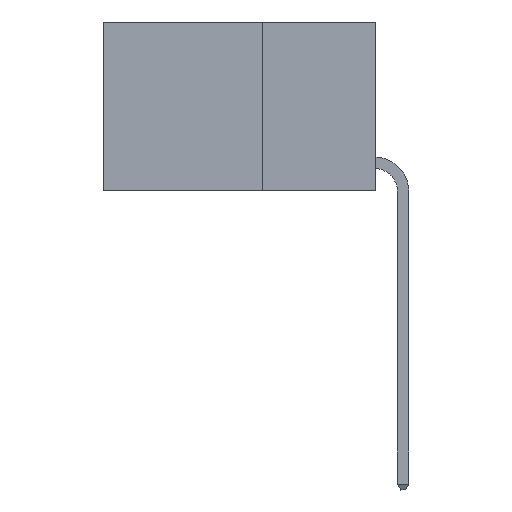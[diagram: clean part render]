
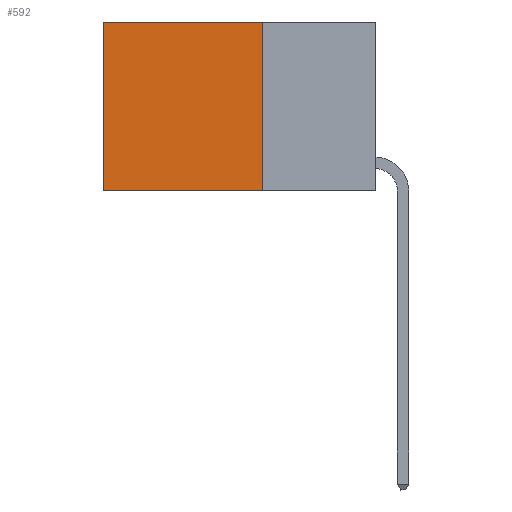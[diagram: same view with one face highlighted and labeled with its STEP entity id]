
A CAD part, left-side view. The second image highlights one B-rep face of the part: STEP entity #592.
In plain terms, the highlighted planar face has unit normal (-1, 0, 0).
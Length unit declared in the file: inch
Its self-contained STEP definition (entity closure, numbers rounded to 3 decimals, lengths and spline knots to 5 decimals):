
#522 = CARTESIAN_POINT ( 'NONE',  ( 0.2625, 0.6, -0.37 ) ) ;
#592 = ADVANCED_FACE ( 'NONE', ( #8254 ), #10887, .F. ) ;
#2098 = DIRECTION ( 'NONE',  ( 0., 0., -1. ) ) ;
#2236 = CARTESIAN_POINT ( 'NONE',  ( 0.2625, 0.6, 0. ) ) ;
#2284 = CARTESIAN_POINT ( 'NONE',  ( 0.2625, 0.25, 0. ) ) ;
#2409 = EDGE_LOOP ( 'NONE', ( #10118, #5816, #7490, #9501 ) ) ;
#2609 = CARTESIAN_POINT ( 'NONE',  ( 0.2625, 0.25, 0. ) ) ;
#2735 = VECTOR ( 'NONE', #2098, 39.37008 ) ;
#3269 = VERTEX_POINT ( 'NONE', #522 ) ;
#4774 = CARTESIAN_POINT ( 'NONE',  ( 0.2625, 0.25, -0.37 ) ) ;
#4839 = EDGE_CURVE ( 'NONE', #11436, #3269, #16387, .T. ) ;
#5131 = CARTESIAN_POINT ( 'NONE',  ( 0.2625, 0.25, 0. ) ) ;
#5227 = DIRECTION ( 'NONE',  ( 0., 0., -1. ) ) ;
#5327 = CARTESIAN_POINT ( 'NONE',  ( 0.2625, 0.6, 0. ) ) ;
#5699 = CARTESIAN_POINT ( 'NONE',  ( 0.2625, 0.25, -0.37 ) ) ;
#5816 = ORIENTED_EDGE ( 'NONE', *, *, #4839, .F. ) ;
#6326 = EDGE_CURVE ( 'NONE', #12104, #16084, #16906, .T. ) ;
#6970 = VECTOR ( 'NONE', #11601, 39.37008 ) ;
#7424 = VECTOR ( 'NONE', #14288, 39.37008 ) ;
#7490 = ORIENTED_EDGE ( 'NONE', *, *, #15593, .F. ) ;
#8254 = FACE_OUTER_BOUND ( 'NONE', #2409, .T. ) ;
#8407 = AXIS2_PLACEMENT_3D ( 'NONE', #2609, #16117, #16286 ) ;
#8948 = LINE ( 'NONE', #2236, #9751 ) ;
#9501 = ORIENTED_EDGE ( 'NONE', *, *, #6326, .T. ) ;
#9751 = VECTOR ( 'NONE', #5227, 39.37008 ) ;
#10118 = ORIENTED_EDGE ( 'NONE', *, *, #15272, .T. ) ;
#10236 = LINE ( 'NONE', #2284, #2735 ) ;
#10529 = CARTESIAN_POINT ( 'NONE',  ( 0.2625, 0.25, 0. ) ) ;
#10887 = PLANE ( 'NONE',  #8407 ) ;
#11436 = VERTEX_POINT ( 'NONE', #5699 ) ;
#11601 = DIRECTION ( 'NONE',  ( 0., 1., 0. ) ) ;
#12104 = VERTEX_POINT ( 'NONE', #5131 ) ;
#14288 = DIRECTION ( 'NONE',  ( 0., 1., 0. ) ) ;
#15272 = EDGE_CURVE ( 'NONE', #16084, #3269, #8948, .T. ) ;
#15593 = EDGE_CURVE ( 'NONE', #12104, #11436, #10236, .T. ) ;
#16084 = VERTEX_POINT ( 'NONE', #5327 ) ;
#16117 = DIRECTION ( 'NONE',  ( 1., 0., 0. ) ) ;
#16286 = DIRECTION ( 'NONE',  ( 0., 0., -1. ) ) ;
#16387 = LINE ( 'NONE', #4774, #7424 ) ;
#16906 = LINE ( 'NONE', #10529, #6970 ) ;
